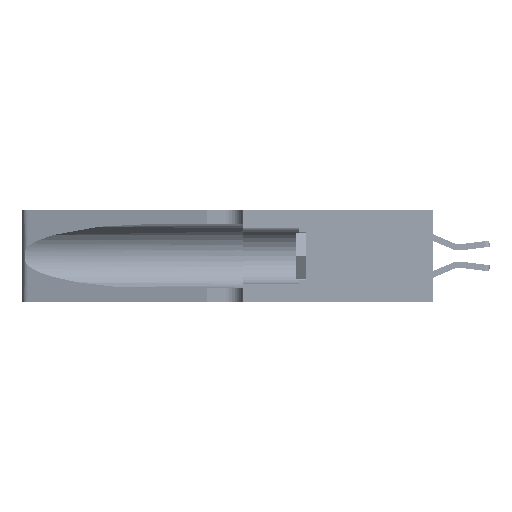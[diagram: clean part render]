
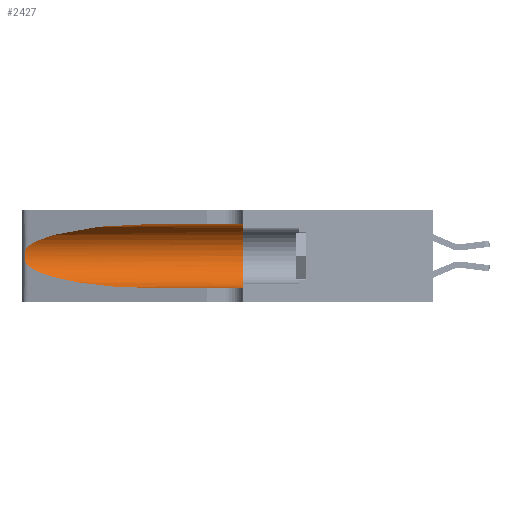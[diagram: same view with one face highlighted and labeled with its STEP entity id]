
A CAD part, left-side view. The second image highlights one B-rep face of the part: STEP entity #2427.
In plain terms, the highlighted cylindrical face has radius 3.308 mm (diameter 6.617 mm), a partial arc.
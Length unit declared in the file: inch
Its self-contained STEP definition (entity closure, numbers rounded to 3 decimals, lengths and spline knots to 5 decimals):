
#2127 = CARTESIAN_POINT ( 'NONE',  ( 0.2373, 1.15595, 0.08982 ) ) ;
#2146 = CARTESIAN_POINT ( 'NONE',  ( 0.25487, 1.22718, 0.22369 ) ) ;
#2280 = CARTESIAN_POINT ( 'NONE',  ( 0.25487, 1.22718, 0.14631 ) ) ;
#2427 = ADVANCED_FACE ( 'NONE', ( #9341 ), #32700, .F. ) ;
#2695 = LINE ( 'NONE', #11097, #18228 ) ;
#3493 = AXIS2_PLACEMENT_3D ( 'NONE', #22208, #3715, #9954 ) ;
#3546 = CIRCLE ( 'NONE', #32802, 0.13025 ) ;
#3715 = DIRECTION ( 'NONE',  ( 0., -1., 0. ) ) ;
#3852 = CARTESIAN_POINT ( 'NONE',  ( 0.1305, 0.35, 0.05475 ) ) ;
#3995 = CARTESIAN_POINT ( 'NONE',  ( 0.1305, 0.72297, 0.31525 ) ) ;
#4041 = VERTEX_POINT ( 'NONE', #4574 ) ;
#4133 = ORIENTED_EDGE ( 'NONE', *, *, #36501, .F. ) ;
#4574 = CARTESIAN_POINT ( 'NONE',  ( 0.25487, 1.22718, 0.22369 ) ) ;
#4951 =( BOUNDED_CURVE ( )  B_SPLINE_CURVE ( 3, ( #20689, #2127, #23704, #5275 ),
 .UNSPECIFIED., .F., .T. ) 
 B_SPLINE_CURVE_WITH_KNOTS ( ( 4, 4 ),
 ( 3.44316, 4.71239 ),
 .UNSPECIFIED. ) 
 CURVE ( )  GEOMETRIC_REPRESENTATION_ITEM ( )  RATIONAL_B_SPLINE_CURVE ( ( 1., 0.87, 0.87, 1. ) ) 
 REPRESENTATION_ITEM ( '' )  );
#5275 = CARTESIAN_POINT ( 'NONE',  ( 0.1305, 0.72297, 0.05475 ) ) ;
#5297 = CARTESIAN_POINT ( 'NONE',  ( 0.25639, 1.23184, 0.21858 ) ) ;
#6292 = CARTESIAN_POINT ( 'NONE',  ( 0.1305, 0.35, 0.31525 ) ) ;
#6705 = ORIENTED_EDGE ( 'NONE', *, *, #22702, .T. ) ;
#7107 = CARTESIAN_POINT ( 'NONE',  ( 0.2373, 1.15595, 0.28018 ) ) ;
#7350 = B_SPLINE_CURVE_WITH_KNOTS ( 'NONE', 3,
 ( #2146, #23724, #5297, #26795, #8410, #29802, #11564, #32825, #14688, #35805, #17769, #38795, #20840, #2280 ),
 .UNSPECIFIED., .F., .F.,
 ( 4, 2, 2, 2, 2, 2, 4 ),
 ( 0., 0.00027, 0.00053, 0.00107, 0.0016, 0.00187, 0.00214 ),
 .UNSPECIFIED. ) ;
#7944 = DIRECTION ( 'NONE',  ( 0., -1., 0. ) ) ;
#8067 = EDGE_CURVE ( 'NONE', #38356, #4041, #15455, .T. ) ;
#8160 = DIRECTION ( 'NONE',  ( 0., 1., 0. ) ) ;
#8410 = CARTESIAN_POINT ( 'NONE',  ( 0.25854, 1.2359, 0.20912 ) ) ;
#8458 = VERTEX_POINT ( 'NONE', #6292 ) ;
#9341 = FACE_OUTER_BOUND ( 'NONE', #24981, .T. ) ;
#9954 = DIRECTION ( 'NONE',  ( 0., 0., -1. ) ) ;
#9998 = VERTEX_POINT ( 'NONE', #20684 ) ;
#10546 = EDGE_CURVE ( 'NONE', #37138, #19603, #2695, .T. ) ;
#11097 = CARTESIAN_POINT ( 'NONE',  ( 0.1305, 1.61858, 0.05475 ) ) ;
#11564 = CARTESIAN_POINT ( 'NONE',  ( 0.26075, 1.23896, 0.19203 ) ) ;
#12824 = EDGE_CURVE ( 'NONE', #8458, #19603, #3546, .T. ) ;
#14688 = CARTESIAN_POINT ( 'NONE',  ( 0.26017, 1.23833, 0.17102 ) ) ;
#15455 =( BOUNDED_CURVE ( )  B_SPLINE_CURVE ( 3, ( #3995, #22469, #7107, #28561 ),
 .UNSPECIFIED., .F., .T. ) 
 B_SPLINE_CURVE_WITH_KNOTS ( ( 4, 4 ),
 ( 1.5708, 2.84003 ),
 .UNSPECIFIED. ) 
 CURVE ( )  GEOMETRIC_REPRESENTATION_ITEM ( )  RATIONAL_B_SPLINE_CURVE ( ( 1., 0.87, 0.87, 1. ) ) 
 REPRESENTATION_ITEM ( '' )  );
#16052 = DIRECTION ( 'NONE',  ( 0., -1., 0. ) ) ;
#16320 = ORIENTED_EDGE ( 'NONE', *, *, #10546, .T. ) ;
#17499 = VECTOR ( 'NONE', #16052, 39.37008 ) ;
#17769 = CARTESIAN_POINT ( 'NONE',  ( 0.25789, 1.23486, 0.15765 ) ) ;
#17986 = EDGE_CURVE ( 'NONE', #4041, #9998, #7350, .T. ) ;
#18228 = VECTOR ( 'NONE', #7944, 39.37008 ) ;
#18465 = LINE ( 'NONE', #31148, #17499 ) ;
#19603 = VERTEX_POINT ( 'NONE', #3852 ) ;
#20684 = CARTESIAN_POINT ( 'NONE',  ( 0.25487, 1.22718, 0.14631 ) ) ;
#20689 = CARTESIAN_POINT ( 'NONE',  ( 0.25487, 1.22718, 0.14631 ) ) ;
#20840 = CARTESIAN_POINT ( 'NONE',  ( 0.25555, 1.22993, 0.14849 ) ) ;
#22208 = CARTESIAN_POINT ( 'NONE',  ( 0.1305, 1.61858, 0.185 ) ) ;
#22469 = CARTESIAN_POINT ( 'NONE',  ( 0.18966, 0.96281, 0.31525 ) ) ;
#22702 = EDGE_CURVE ( 'NONE', #9998, #37138, #4951, .T. ) ;
#22740 = ORIENTED_EDGE ( 'NONE', *, *, #8067, .T. ) ;
#23704 = CARTESIAN_POINT ( 'NONE',  ( 0.18966, 0.96281, 0.05475 ) ) ;
#23724 = CARTESIAN_POINT ( 'NONE',  ( 0.25555, 1.22994, 0.2215 ) ) ;
#24411 = CARTESIAN_POINT ( 'NONE',  ( 0.1305, 0.72297, 0.31525 ) ) ;
#24981 = EDGE_LOOP ( 'NONE', ( #22740, #33095, #6705, #16320, #24990, #4133 ) ) ;
#24990 = ORIENTED_EDGE ( 'NONE', *, *, #12824, .F. ) ;
#26540 = CARTESIAN_POINT ( 'NONE',  ( 0.1305, 0.35, 0.185 ) ) ;
#26795 = CARTESIAN_POINT ( 'NONE',  ( 0.25787, 1.23484, 0.2124 ) ) ;
#28561 = CARTESIAN_POINT ( 'NONE',  ( 0.25487, 1.22718, 0.22369 ) ) ;
#29571 = DIRECTION ( 'NONE',  ( 0., 0., 1. ) ) ;
#29802 = CARTESIAN_POINT ( 'NONE',  ( 0.26018, 1.23835, 0.19895 ) ) ;
#31148 = CARTESIAN_POINT ( 'NONE',  ( 0.1305, 1.61858, 0.31525 ) ) ;
#32700 = CYLINDRICAL_SURFACE ( 'NONE', #3493, 0.13025 ) ;
#32802 = AXIS2_PLACEMENT_3D ( 'NONE', #26540, #8160, #29571 ) ;
#32825 = CARTESIAN_POINT ( 'NONE',  ( 0.26075, 1.23896, 0.178 ) ) ;
#33095 = ORIENTED_EDGE ( 'NONE', *, *, #17986, .T. ) ;
#34117 = CARTESIAN_POINT ( 'NONE',  ( 0.1305, 0.72297, 0.05475 ) ) ;
#35805 = CARTESIAN_POINT ( 'NONE',  ( 0.25856, 1.23593, 0.16098 ) ) ;
#36501 = EDGE_CURVE ( 'NONE', #38356, #8458, #18465, .T. ) ;
#37138 = VERTEX_POINT ( 'NONE', #34117 ) ;
#38356 = VERTEX_POINT ( 'NONE', #24411 ) ;
#38795 = CARTESIAN_POINT ( 'NONE',  ( 0.25639, 1.23186, 0.15144 ) ) ;
